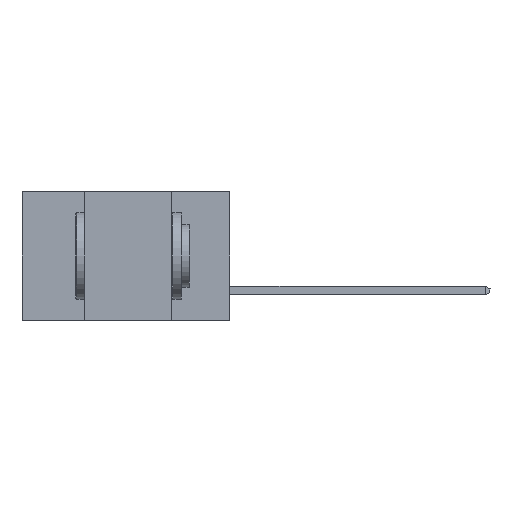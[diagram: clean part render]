
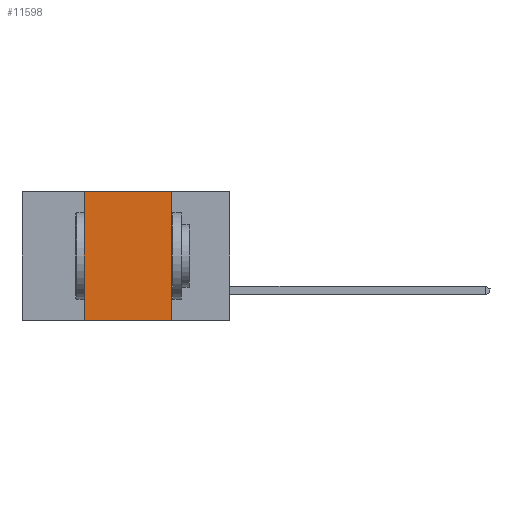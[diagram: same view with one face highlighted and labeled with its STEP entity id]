
A CAD part, left-side view. The second image highlights one B-rep face of the part: STEP entity #11598.
In plain terms, the highlighted planar face has unit normal (-1, 0, 0).
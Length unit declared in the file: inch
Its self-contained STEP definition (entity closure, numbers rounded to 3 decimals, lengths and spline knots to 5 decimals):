
#126 = VERTEX_POINT ( 'NONE', #2850 ) ;
#239 = DIRECTION ( 'NONE',  ( 0., 0., 1. ) ) ;
#650 = CARTESIAN_POINT ( 'NONE',  ( 0., 0.17, -0.37 ) ) ;
#937 = DIRECTION ( 'NONE',  ( 0., 0., -1. ) ) ;
#1122 = ORIENTED_EDGE ( 'NONE', *, *, #13120, .F. ) ;
#1260 = EDGE_CURVE ( 'NONE', #126, #8945, #14762, .T. ) ;
#2283 = DIRECTION ( 'NONE',  ( 1., 0., 0. ) ) ;
#2850 = CARTESIAN_POINT ( 'NONE',  ( 0., 0.17, 0. ) ) ;
#2871 = LINE ( 'NONE', #13981, #8656 ) ;
#3658 = VERTEX_POINT ( 'NONE', #10112 ) ;
#3887 = DIRECTION ( 'NONE',  ( 0., 0., -1. ) ) ;
#3893 = CARTESIAN_POINT ( 'NONE',  ( 0., 0.6, 0. ) ) ;
#3980 = EDGE_CURVE ( 'NONE', #3658, #10525, #7552, .T. ) ;
#4171 = VECTOR ( 'NONE', #3887, 39.37008 ) ;
#4603 = VECTOR ( 'NONE', #11571, 39.37008 ) ;
#4731 = EDGE_LOOP ( 'NONE', ( #10923, #1122, #8427, #12982 ) ) ;
#5162 = LINE ( 'NONE', #3893, #4603 ) ;
#5409 = DIRECTION ( 'NONE',  ( 0., -1., 0. ) ) ;
#7552 = LINE ( 'NONE', #12634, #12300 ) ;
#8427 = ORIENTED_EDGE ( 'NONE', *, *, #3980, .F. ) ;
#8656 = VECTOR ( 'NONE', #5409, 39.37008 ) ;
#8945 = VERTEX_POINT ( 'NONE', #650 ) ;
#10112 = CARTESIAN_POINT ( 'NONE',  ( 0., 0.42, -0.37 ) ) ;
#10525 = VERTEX_POINT ( 'NONE', #14504 ) ;
#10532 = CARTESIAN_POINT ( 'NONE',  ( 0., 0.6, 0. ) ) ;
#10923 = ORIENTED_EDGE ( 'NONE', *, *, #1260, .F. ) ;
#11571 = DIRECTION ( 'NONE',  ( 0., -1., 0. ) ) ;
#11598 = ADVANCED_FACE ( 'NONE', ( #15542 ), #11812, .F. ) ;
#11812 = PLANE ( 'NONE',  #12433 ) ;
#12300 = VECTOR ( 'NONE', #239, 39.37008 ) ;
#12433 = AXIS2_PLACEMENT_3D ( 'NONE', #10532, #2283, #937 ) ;
#12634 = CARTESIAN_POINT ( 'NONE',  ( 0., 0.42, -0.37 ) ) ;
#12982 = ORIENTED_EDGE ( 'NONE', *, *, #15111, .T. ) ;
#13120 = EDGE_CURVE ( 'NONE', #10525, #126, #5162, .T. ) ;
#13577 = CARTESIAN_POINT ( 'NONE',  ( 0., 0.17, -0.37 ) ) ;
#13981 = CARTESIAN_POINT ( 'NONE',  ( 0., 0.6, -0.37 ) ) ;
#14504 = CARTESIAN_POINT ( 'NONE',  ( 0., 0.42, 0. ) ) ;
#14762 = LINE ( 'NONE', #13577, #4171 ) ;
#15111 = EDGE_CURVE ( 'NONE', #3658, #8945, #2871, .T. ) ;
#15542 = FACE_OUTER_BOUND ( 'NONE', #4731, .T. ) ;
